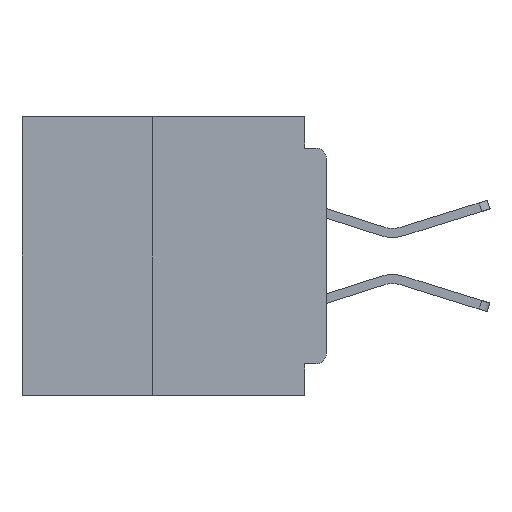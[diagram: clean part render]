
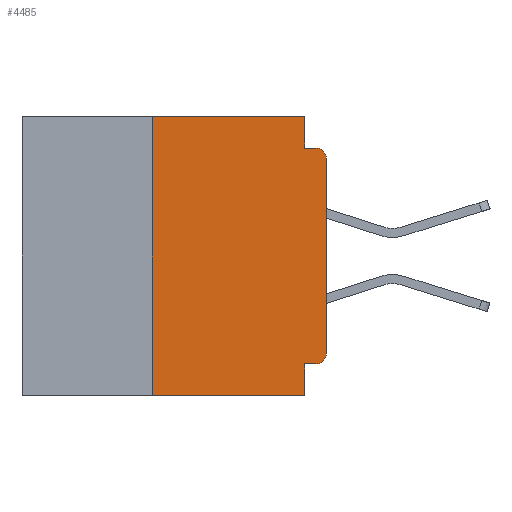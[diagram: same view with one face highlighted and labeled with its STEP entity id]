
A CAD part, left-side view. The second image highlights one B-rep face of the part: STEP entity #4485.
In plain terms, the highlighted planar face has unit normal (-1, 0, 0).
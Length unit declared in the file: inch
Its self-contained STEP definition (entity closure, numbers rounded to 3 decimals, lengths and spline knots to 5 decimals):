
#82 = VERTEX_POINT ( 'NONE', #41886 ) ;
#798 = ORIENTED_EDGE ( 'NONE', *, *, #1917, .F. ) ;
#1578 = VECTOR ( 'NONE', #40223, 39.37008 ) ;
#1917 = EDGE_CURVE ( 'NONE', #82, #13917, #50595, .T. ) ;
#1933 = CIRCLE ( 'NONE', #23158, 0.015 ) ;
#2146 = DIRECTION ( 'NONE',  ( 0., 0., -1. ) ) ;
#2844 = CARTESIAN_POINT ( 'NONE',  ( 0., 0.25, -0.4 ) ) ;
#4485 = ADVANCED_FACE ( 'NONE', ( #4954 ), #22119, .F. ) ;
#4826 = DIRECTION ( 'NONE',  ( 0., 0., 1. ) ) ;
#4954 = FACE_OUTER_BOUND ( 'NONE', #5952, .T. ) ;
#5952 = EDGE_LOOP ( 'NONE', ( #55919, #49676, #798, #26524, #42718, #48325, #9441, #7357, #34425, #25205 ) ) ;
#6436 = CARTESIAN_POINT ( 'NONE',  ( 0., 0.031, -0.4 ) ) ;
#6543 = LINE ( 'NONE', #46210, #53188 ) ;
#6725 = CARTESIAN_POINT ( 'NONE',  ( 0., 0.015, -0.045 ) ) ;
#7357 = ORIENTED_EDGE ( 'NONE', *, *, #23086, .F. ) ;
#8082 = CIRCLE ( 'NONE', #34423, 0.015 ) ;
#8150 = LINE ( 'NONE', #51743, #54760 ) ;
#8647 = VECTOR ( 'NONE', #4826, 39.37008 ) ;
#9441 = ORIENTED_EDGE ( 'NONE', *, *, #56018, .T. ) ;
#10058 = LINE ( 'NONE', #36415, #8647 ) ;
#11260 = EDGE_CURVE ( 'NONE', #32095, #27800, #24807, .T. ) ;
#11267 = DIRECTION ( 'NONE',  ( 0., 0., -1. ) ) ;
#11313 = CARTESIAN_POINT ( 'NONE',  ( 0., 0.015, -0.06 ) ) ;
#13042 = DIRECTION ( 'NONE',  ( 0., -1., 0. ) ) ;
#13917 = VERTEX_POINT ( 'NONE', #6725 ) ;
#15944 = DIRECTION ( 'NONE',  ( 0., 0., -1. ) ) ;
#16985 = DIRECTION ( 'NONE',  ( -1., 0., 0. ) ) ;
#17285 = EDGE_CURVE ( 'NONE', #27800, #45475, #6543, .T. ) ;
#19215 = DIRECTION ( 'NONE',  ( 0., -1., 0. ) ) ;
#21673 = DIRECTION ( 'NONE',  ( 0., 0., -1. ) ) ;
#21865 = DIRECTION ( 'NONE',  ( 1., 0., 0. ) ) ;
#22056 = CARTESIAN_POINT ( 'NONE',  ( 0., 0.437, 0. ) ) ;
#22119 = PLANE ( 'NONE',  #47402 ) ;
#23086 = EDGE_CURVE ( 'NONE', #23888, #34413, #49259, .T. ) ;
#23158 = AXIS2_PLACEMENT_3D ( 'NONE', #44017, #16985, #48508 ) ;
#23214 = CARTESIAN_POINT ( 'NONE',  ( 0., 0., -0.34 ) ) ;
#23528 = VERTEX_POINT ( 'NONE', #46125 ) ;
#23888 = VERTEX_POINT ( 'NONE', #39187 ) ;
#24807 = LINE ( 'NONE', #26140, #56350 ) ;
#25205 = ORIENTED_EDGE ( 'NONE', *, *, #50975, .T. ) ;
#26140 = CARTESIAN_POINT ( 'NONE',  ( 0., 0.25, -0.4 ) ) ;
#26524 = ORIENTED_EDGE ( 'NONE', *, *, #52825, .F. ) ;
#27233 = EDGE_CURVE ( 'NONE', #23528, #23888, #49786, .T. ) ;
#27800 = VERTEX_POINT ( 'NONE', #48595 ) ;
#27994 = EDGE_CURVE ( 'NONE', #53224, #51759, #10058, .T. ) ;
#28009 = VECTOR ( 'NONE', #13042, 39.37008 ) ;
#29427 = LINE ( 'NONE', #35682, #28009 ) ;
#30328 = CARTESIAN_POINT ( 'NONE',  ( 0., 0., -0.045 ) ) ;
#31351 = EDGE_CURVE ( 'NONE', #51759, #13917, #8082, .T. ) ;
#32095 = VERTEX_POINT ( 'NONE', #2844 ) ;
#33117 = DIRECTION ( 'NONE',  ( 0., -1., 0. ) ) ;
#34413 = VERTEX_POINT ( 'NONE', #6436 ) ;
#34423 = AXIS2_PLACEMENT_3D ( 'NONE', #11313, #43012, #15944 ) ;
#34425 = ORIENTED_EDGE ( 'NONE', *, *, #27233, .F. ) ;
#35682 = CARTESIAN_POINT ( 'NONE',  ( 0., 0.437, -0.4 ) ) ;
#36415 = CARTESIAN_POINT ( 'NONE',  ( 0., 0., 0. ) ) ;
#37280 = VECTOR ( 'NONE', #33117, 39.37008 ) ;
#39187 = CARTESIAN_POINT ( 'NONE',  ( 0., 0.031, -0.355 ) ) ;
#40223 = DIRECTION ( 'NONE',  ( 0., 1., 0. ) ) ;
#41886 = CARTESIAN_POINT ( 'NONE',  ( 0., 0.031, -0.045 ) ) ;
#42718 = ORIENTED_EDGE ( 'NONE', *, *, #17285, .F. ) ;
#43012 = DIRECTION ( 'NONE',  ( -1., 0., 0. ) ) ;
#43050 = CARTESIAN_POINT ( 'NONE',  ( 0., 0.031, -0.4 ) ) ;
#44017 = CARTESIAN_POINT ( 'NONE',  ( 0., 0.015, -0.34 ) ) ;
#44037 = DIRECTION ( 'NONE',  ( 0., 0., 1. ) ) ;
#45392 = CARTESIAN_POINT ( 'NONE',  ( 0., 0.031, 0. ) ) ;
#45475 = VERTEX_POINT ( 'NONE', #45392 ) ;
#46125 = CARTESIAN_POINT ( 'NONE',  ( 0., 0.015, -0.355 ) ) ;
#46210 = CARTESIAN_POINT ( 'NONE',  ( 0., 0.437, 0. ) ) ;
#47402 = AXIS2_PLACEMENT_3D ( 'NONE', #22056, #21865, #21673 ) ;
#48325 = ORIENTED_EDGE ( 'NONE', *, *, #11260, .F. ) ;
#48508 = DIRECTION ( 'NONE',  ( 0., 0., -1. ) ) ;
#48595 = CARTESIAN_POINT ( 'NONE',  ( 0., 0.25, 0. ) ) ;
#49259 = LINE ( 'NONE', #43050, #58259 ) ;
#49676 = ORIENTED_EDGE ( 'NONE', *, *, #31351, .T. ) ;
#49786 = LINE ( 'NONE', #57950, #1578 ) ;
#50595 = LINE ( 'NONE', #30328, #37280 ) ;
#50975 = EDGE_CURVE ( 'NONE', #23528, #53224, #1933, .T. ) ;
#51743 = CARTESIAN_POINT ( 'NONE',  ( 0., 0.031, 0. ) ) ;
#51759 = VERTEX_POINT ( 'NONE', #54663 ) ;
#52825 = EDGE_CURVE ( 'NONE', #45475, #82, #8150, .T. ) ;
#53188 = VECTOR ( 'NONE', #19215, 39.37008 ) ;
#53224 = VERTEX_POINT ( 'NONE', #23214 ) ;
#54663 = CARTESIAN_POINT ( 'NONE',  ( 0., 0., -0.06 ) ) ;
#54760 = VECTOR ( 'NONE', #11267, 39.37008 ) ;
#55919 = ORIENTED_EDGE ( 'NONE', *, *, #27994, .T. ) ;
#56018 = EDGE_CURVE ( 'NONE', #32095, #34413, #29427, .T. ) ;
#56350 = VECTOR ( 'NONE', #44037, 39.37008 ) ;
#57950 = CARTESIAN_POINT ( 'NONE',  ( 0., 0., -0.355 ) ) ;
#58259 = VECTOR ( 'NONE', #2146, 39.37008 ) ;
